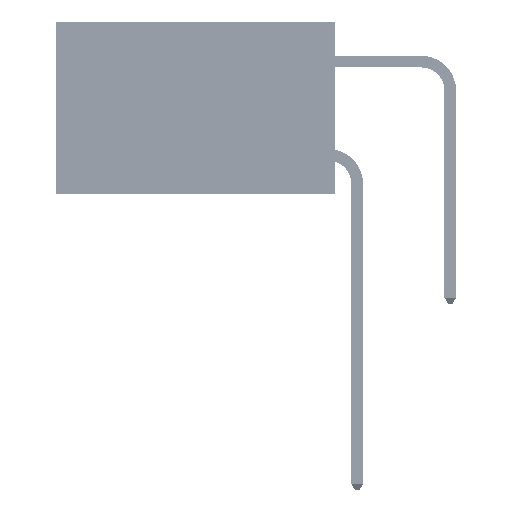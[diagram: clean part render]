
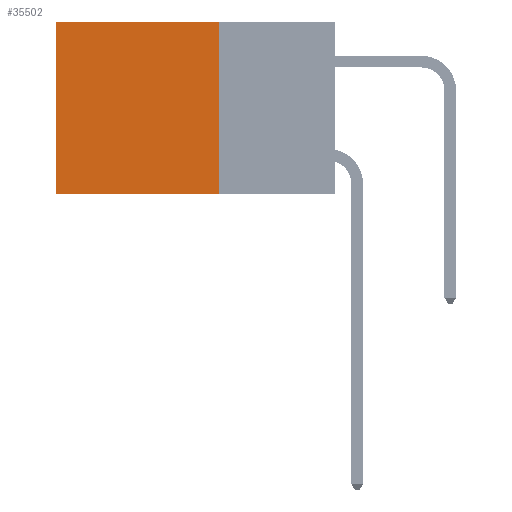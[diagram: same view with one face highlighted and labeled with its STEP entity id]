
A CAD part, left-side view. The second image highlights one B-rep face of the part: STEP entity #35502.
In plain terms, the highlighted planar face has unit normal (-1, 0, 0).
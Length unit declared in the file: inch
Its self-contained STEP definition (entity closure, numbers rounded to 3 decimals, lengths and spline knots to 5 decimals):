
#659 = ORIENTED_EDGE ( 'NONE', *, *, #5131, .F. ) ;
#1889 = EDGE_LOOP ( 'NONE', ( #7608, #43497, #659, #27313 ) ) ;
#5131 = EDGE_CURVE ( 'NONE', #45975, #41550, #7618, .T. ) ;
#5658 = AXIS2_PLACEMENT_3D ( 'NONE', #23409, #39749, #15392 ) ;
#5961 = VERTEX_POINT ( 'NONE', #49300 ) ;
#6894 = EDGE_CURVE ( 'NONE', #7281, #5961, #21610, .T. ) ;
#7281 = VERTEX_POINT ( 'NONE', #13363 ) ;
#7556 = LINE ( 'NONE', #24343, #17195 ) ;
#7608 = ORIENTED_EDGE ( 'NONE', *, *, #6894, .T. ) ;
#7618 = LINE ( 'NONE', #23885, #38875 ) ;
#7811 = LINE ( 'NONE', #18848, #39066 ) ;
#11039 = CARTESIAN_POINT ( 'NONE',  ( 0.2875, 0.6, 0. ) ) ;
#13363 = CARTESIAN_POINT ( 'NONE',  ( 0.2875, 0.6, 0. ) ) ;
#15392 = DIRECTION ( 'NONE',  ( 0., 0., -1. ) ) ;
#17195 = VECTOR ( 'NONE', #44701, 39.37008 ) ;
#18848 = CARTESIAN_POINT ( 'NONE',  ( 0.2875, 0.25, 0. ) ) ;
#21610 = LINE ( 'NONE', #11039, #33706 ) ;
#22938 = DIRECTION ( 'NONE',  ( 0., 1., 0. ) ) ;
#23409 = CARTESIAN_POINT ( 'NONE',  ( 0.2875, 0.25, 0. ) ) ;
#23885 = CARTESIAN_POINT ( 'NONE',  ( 0.2875, 0.25, 0. ) ) ;
#24343 = CARTESIAN_POINT ( 'NONE',  ( 0.2875, 0.25, -0.37 ) ) ;
#27313 = ORIENTED_EDGE ( 'NONE', *, *, #36742, .T. ) ;
#27846 = FACE_OUTER_BOUND ( 'NONE', #1889, .T. ) ;
#31110 = CARTESIAN_POINT ( 'NONE',  ( 0.2875, 0.25, -0.37 ) ) ;
#32061 = DIRECTION ( 'NONE',  ( 0., 0., -1. ) ) ;
#33706 = VECTOR ( 'NONE', #39535, 39.37008 ) ;
#35502 = ADVANCED_FACE ( 'NONE', ( #27846 ), #35675, .F. ) ;
#35675 = PLANE ( 'NONE',  #5658 ) ;
#36742 = EDGE_CURVE ( 'NONE', #45975, #7281, #7811, .T. ) ;
#38875 = VECTOR ( 'NONE', #32061, 39.37008 ) ;
#38983 = EDGE_CURVE ( 'NONE', #41550, #5961, #7556, .T. ) ;
#39066 = VECTOR ( 'NONE', #22938, 39.37008 ) ;
#39248 = CARTESIAN_POINT ( 'NONE',  ( 0.2875, 0.25, 0. ) ) ;
#39535 = DIRECTION ( 'NONE',  ( 0., 0., -1. ) ) ;
#39749 = DIRECTION ( 'NONE',  ( 1., 0., 0. ) ) ;
#41550 = VERTEX_POINT ( 'NONE', #31110 ) ;
#43497 = ORIENTED_EDGE ( 'NONE', *, *, #38983, .F. ) ;
#44701 = DIRECTION ( 'NONE',  ( 0., 1., 0. ) ) ;
#45975 = VERTEX_POINT ( 'NONE', #39248 ) ;
#49300 = CARTESIAN_POINT ( 'NONE',  ( 0.2875, 0.6, -0.37 ) ) ;
